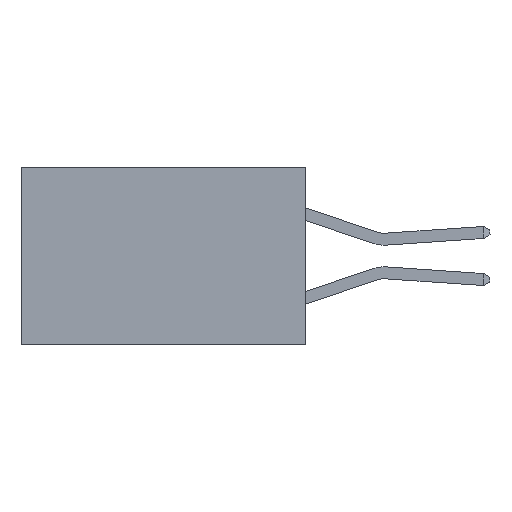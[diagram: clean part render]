
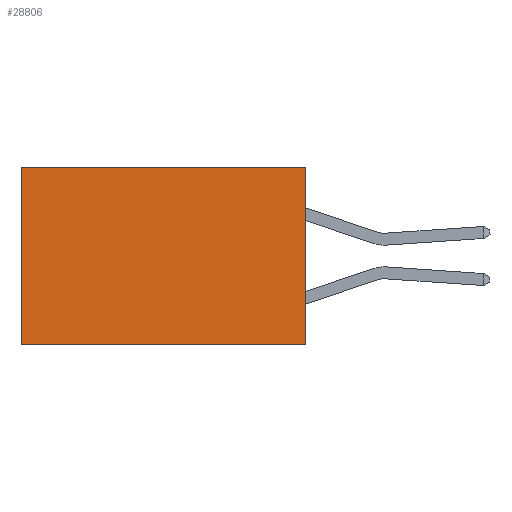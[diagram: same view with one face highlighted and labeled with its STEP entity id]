
A CAD part, left-side view. The second image highlights one B-rep face of the part: STEP entity #28806.
In plain terms, the highlighted planar face has unit normal (-1, 0, 0).
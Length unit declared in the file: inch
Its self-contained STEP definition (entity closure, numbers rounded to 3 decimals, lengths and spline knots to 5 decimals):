
#48 = ORIENTED_EDGE ( 'NONE', *, *, #29982, .F. ) ;
#1041 = VECTOR ( 'NONE', #17614, 39.37008 ) ;
#2361 = VERTEX_POINT ( 'NONE', #7133 ) ;
#3218 = VECTOR ( 'NONE', #10989, 39.37008 ) ;
#4254 = EDGE_CURVE ( 'NONE', #2361, #29702, #22750, .T. ) ;
#4824 = CARTESIAN_POINT ( 'NONE',  ( 0.277, 0.59, -0.37 ) ) ;
#5752 = ORIENTED_EDGE ( 'NONE', *, *, #23946, .F. ) ;
#5911 = LINE ( 'NONE', #21226, #19522 ) ;
#7133 = CARTESIAN_POINT ( 'NONE',  ( 0.277, 0., 0. ) ) ;
#7709 = DIRECTION ( 'NONE',  ( 0., 1., 0. ) ) ;
#8076 = PLANE ( 'NONE',  #19894 ) ;
#8242 = CARTESIAN_POINT ( 'NONE',  ( 0.277, 0., -0.37 ) ) ;
#10989 = DIRECTION ( 'NONE',  ( 0., 0., -1. ) ) ;
#13050 = DIRECTION ( 'NONE',  ( 0., 0., -1. ) ) ;
#13531 = DIRECTION ( 'NONE',  ( 0., 0., -1. ) ) ;
#15154 = CARTESIAN_POINT ( 'NONE',  ( 0.277, 0.59, 0. ) ) ;
#17614 = DIRECTION ( 'NONE',  ( 0., 1., 0. ) ) ;
#17700 = LINE ( 'NONE', #8242, #3218 ) ;
#19097 = CARTESIAN_POINT ( 'NONE',  ( 0.277, 0., 0. ) ) ;
#19522 = VECTOR ( 'NONE', #7709, 39.37008 ) ;
#19894 = AXIS2_PLACEMENT_3D ( 'NONE', #26994, #29693, #13531 ) ;
#21154 = EDGE_CURVE ( 'NONE', #29702, #30928, #30180, .T. ) ;
#21226 = CARTESIAN_POINT ( 'NONE',  ( 0.277, 0., -0.37 ) ) ;
#22400 = EDGE_LOOP ( 'NONE', ( #32568, #5752, #48, #23555 ) ) ;
#22750 = LINE ( 'NONE', #19097, #1041 ) ;
#23555 = ORIENTED_EDGE ( 'NONE', *, *, #4254, .T. ) ;
#23946 = EDGE_CURVE ( 'NONE', #26757, #30928, #5911, .T. ) ;
#26201 = FACE_OUTER_BOUND ( 'NONE', #22400, .T. ) ;
#26757 = VERTEX_POINT ( 'NONE', #27684 ) ;
#26994 = CARTESIAN_POINT ( 'NONE',  ( 0.277, 0., -0.37 ) ) ;
#27684 = CARTESIAN_POINT ( 'NONE',  ( 0.277, 0., -0.37 ) ) ;
#28530 = VECTOR ( 'NONE', #13050, 39.37008 ) ;
#28806 = ADVANCED_FACE ( 'NONE', ( #26201 ), #8076, .F. ) ;
#29693 = DIRECTION ( 'NONE',  ( 1., 0., 0. ) ) ;
#29702 = VERTEX_POINT ( 'NONE', #15154 ) ;
#29982 = EDGE_CURVE ( 'NONE', #2361, #26757, #17700, .T. ) ;
#30180 = LINE ( 'NONE', #4824, #28530 ) ;
#30741 = CARTESIAN_POINT ( 'NONE',  ( 0.277, 0.59, -0.37 ) ) ;
#30928 = VERTEX_POINT ( 'NONE', #30741 ) ;
#32568 = ORIENTED_EDGE ( 'NONE', *, *, #21154, .T. ) ;
